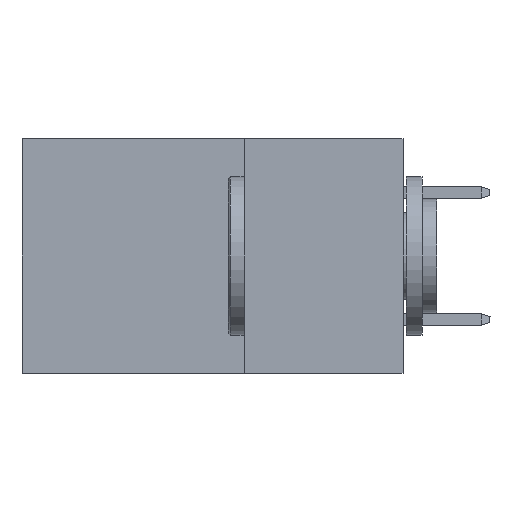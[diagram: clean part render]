
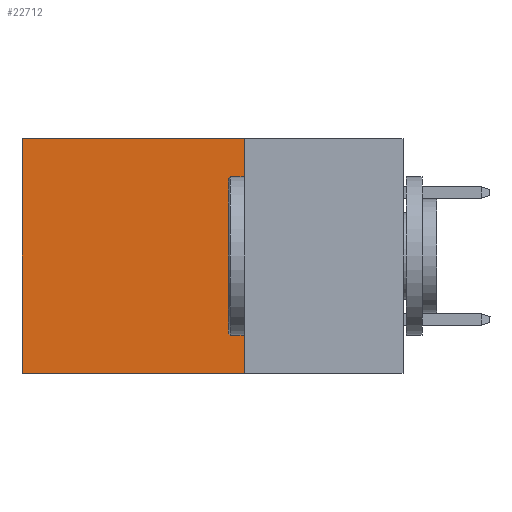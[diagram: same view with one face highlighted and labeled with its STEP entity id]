
A CAD part, left-side view. The second image highlights one B-rep face of the part: STEP entity #22712.
In plain terms, the highlighted planar face has unit normal (-1, 0, 0).
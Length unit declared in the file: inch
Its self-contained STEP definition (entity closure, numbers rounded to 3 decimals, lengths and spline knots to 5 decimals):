
#1550 = VECTOR ( 'NONE', #25375, 39.37008 ) ;
#3128 = LINE ( 'NONE', #20038, #37112 ) ;
#5378 = VERTEX_POINT ( 'NONE', #32285 ) ;
#9218 = ORIENTED_EDGE ( 'NONE', *, *, #30686, .F. ) ;
#11711 = DIRECTION ( 'NONE',  ( 0., 0., -1. ) ) ;
#15044 = CARTESIAN_POINT ( 'NONE',  ( 0.2875, 0.25, 0. ) ) ;
#16217 = CARTESIAN_POINT ( 'NONE',  ( 0.2875, 0.25, 0. ) ) ;
#19470 = FACE_OUTER_BOUND ( 'NONE', #19712, .T. ) ;
#19712 = EDGE_LOOP ( 'NONE', ( #36805, #9218, #33383, #28616 ) ) ;
#20038 = CARTESIAN_POINT ( 'NONE',  ( 0.2875, 0.25, -0.37 ) ) ;
#21060 = VERTEX_POINT ( 'NONE', #38080 ) ;
#21645 = CARTESIAN_POINT ( 'NONE',  ( 0.2875, 0.25, 0. ) ) ;
#21748 = DIRECTION ( 'NONE',  ( 0., 1., 0. ) ) ;
#22712 = ADVANCED_FACE ( 'NONE', ( #19470 ), #32477, .F. ) ;
#24833 = AXIS2_PLACEMENT_3D ( 'NONE', #16217, #29446, #36130 ) ;
#25028 = VECTOR ( 'NONE', #21748, 39.37008 ) ;
#25375 = DIRECTION ( 'NONE',  ( 0., 0., -1. ) ) ;
#27529 = CARTESIAN_POINT ( 'NONE',  ( 0.2875, 0.6, 0. ) ) ;
#28424 = CARTESIAN_POINT ( 'NONE',  ( 0.2875, 0.6, 0. ) ) ;
#28478 = LINE ( 'NONE', #15044, #25028 ) ;
#28616 = ORIENTED_EDGE ( 'NONE', *, *, #36958, .T. ) ;
#29446 = DIRECTION ( 'NONE',  ( 1., 0., 0. ) ) ;
#30686 = EDGE_CURVE ( 'NONE', #5378, #31367, #3128, .T. ) ;
#31196 = LINE ( 'NONE', #21645, #37249 ) ;
#31367 = VERTEX_POINT ( 'NONE', #37694 ) ;
#32285 = CARTESIAN_POINT ( 'NONE',  ( 0.2875, 0.25, -0.37 ) ) ;
#32477 = PLANE ( 'NONE',  #24833 ) ;
#33383 = ORIENTED_EDGE ( 'NONE', *, *, #34882, .F. ) ;
#34882 = EDGE_CURVE ( 'NONE', #21060, #5378, #31196, .T. ) ;
#36130 = DIRECTION ( 'NONE',  ( 0., 0., -1. ) ) ;
#36805 = ORIENTED_EDGE ( 'NONE', *, *, #41878, .T. ) ;
#36958 = EDGE_CURVE ( 'NONE', #21060, #40526, #28478, .T. ) ;
#37112 = VECTOR ( 'NONE', #42574, 39.37008 ) ;
#37249 = VECTOR ( 'NONE', #11711, 39.37008 ) ;
#37694 = CARTESIAN_POINT ( 'NONE',  ( 0.2875, 0.6, -0.37 ) ) ;
#38080 = CARTESIAN_POINT ( 'NONE',  ( 0.2875, 0.25, 0. ) ) ;
#40526 = VERTEX_POINT ( 'NONE', #27529 ) ;
#41878 = EDGE_CURVE ( 'NONE', #40526, #31367, #42053, .T. ) ;
#42053 = LINE ( 'NONE', #28424, #1550 ) ;
#42574 = DIRECTION ( 'NONE',  ( 0., 1., 0. ) ) ;
